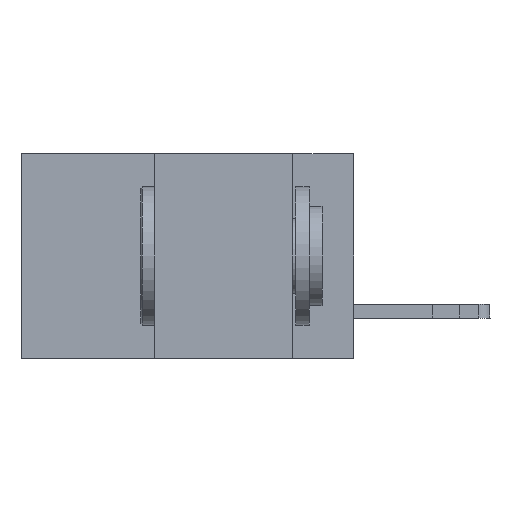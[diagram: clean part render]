
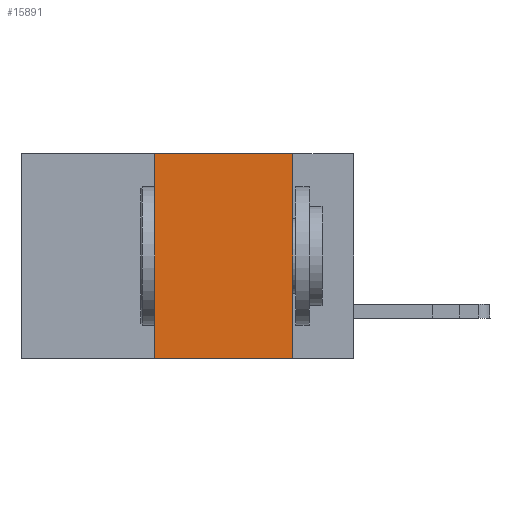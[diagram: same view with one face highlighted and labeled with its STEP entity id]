
A CAD part, left-side view. The second image highlights one B-rep face of the part: STEP entity #15891.
In plain terms, the highlighted planar face has unit normal (-1, 0, 0).
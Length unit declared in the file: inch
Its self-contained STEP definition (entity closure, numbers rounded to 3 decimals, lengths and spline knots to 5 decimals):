
#1745 = LINE ( 'NONE', #26630, #22646 ) ;
#3084 = VERTEX_POINT ( 'NONE', #27297 ) ;
#3290 = ORIENTED_EDGE ( 'NONE', *, *, #23418, .F. ) ;
#3902 = FACE_OUTER_BOUND ( 'NONE', #13473, .T. ) ;
#5265 = DIRECTION ( 'NONE',  ( 0., 0., -1. ) ) ;
#5538 = LINE ( 'NONE', #9256, #23162 ) ;
#5919 = VERTEX_POINT ( 'NONE', #18793 ) ;
#6639 = DIRECTION ( 'NONE',  ( 1., 0., 0. ) ) ;
#7170 = EDGE_CURVE ( 'NONE', #3084, #12588, #1745, .T. ) ;
#7174 = ORIENTED_EDGE ( 'NONE', *, *, #7170, .F. ) ;
#7224 = VECTOR ( 'NONE', #17646, 39.37008 ) ;
#9011 = DIRECTION ( 'NONE',  ( 0., 0., -1. ) ) ;
#9256 = CARTESIAN_POINT ( 'NONE',  ( 0., 0.36, 0. ) ) ;
#10156 = EDGE_CURVE ( 'NONE', #5919, #12588, #25401, .T. ) ;
#11043 = EDGE_CURVE ( 'NONE', #5919, #16935, #5538, .T. ) ;
#11376 = ORIENTED_EDGE ( 'NONE', *, *, #11043, .F. ) ;
#11848 = CARTESIAN_POINT ( 'NONE',  ( 0., 0.6, -0.37 ) ) ;
#12588 = VERTEX_POINT ( 'NONE', #19574 ) ;
#13473 = EDGE_LOOP ( 'NONE', ( #7174, #3290, #11376, #28324 ) ) ;
#14149 = LINE ( 'NONE', #26796, #7224 ) ;
#14676 = AXIS2_PLACEMENT_3D ( 'NONE', #20659, #6639, #9011 ) ;
#15891 = ADVANCED_FACE ( 'NONE', ( #3902 ), #22605, .F. ) ;
#16935 = VERTEX_POINT ( 'NONE', #21439 ) ;
#17646 = DIRECTION ( 'NONE',  ( 0., -1., 0. ) ) ;
#18793 = CARTESIAN_POINT ( 'NONE',  ( 0., 0.36, -0.37 ) ) ;
#19280 = DIRECTION ( 'NONE',  ( 0., -1., 0. ) ) ;
#19574 = CARTESIAN_POINT ( 'NONE',  ( 0., 0.11, -0.37 ) ) ;
#20659 = CARTESIAN_POINT ( 'NONE',  ( 0., 0.6, 0. ) ) ;
#21439 = CARTESIAN_POINT ( 'NONE',  ( 0., 0.36, 0. ) ) ;
#22605 = PLANE ( 'NONE',  #14676 ) ;
#22646 = VECTOR ( 'NONE', #5265, 39.37008 ) ;
#23162 = VECTOR ( 'NONE', #28335, 39.37008 ) ;
#23418 = EDGE_CURVE ( 'NONE', #16935, #3084, #14149, .T. ) ;
#25401 = LINE ( 'NONE', #11848, #28692 ) ;
#26630 = CARTESIAN_POINT ( 'NONE',  ( 0., 0.11, 0. ) ) ;
#26796 = CARTESIAN_POINT ( 'NONE',  ( 0., 0.6, 0. ) ) ;
#27297 = CARTESIAN_POINT ( 'NONE',  ( 0., 0.11, 0. ) ) ;
#28324 = ORIENTED_EDGE ( 'NONE', *, *, #10156, .T. ) ;
#28335 = DIRECTION ( 'NONE',  ( 0., 0., 1. ) ) ;
#28692 = VECTOR ( 'NONE', #19280, 39.37008 ) ;
